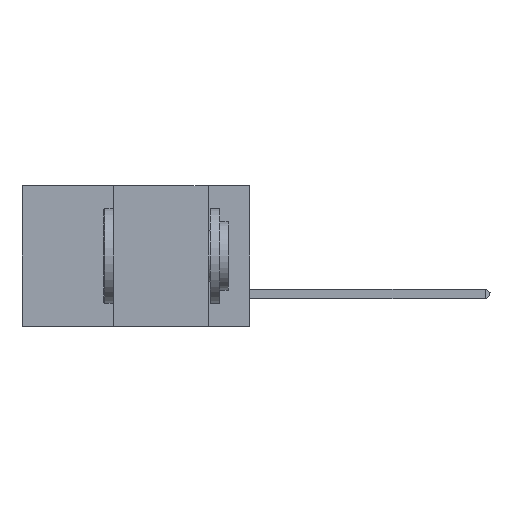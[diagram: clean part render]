
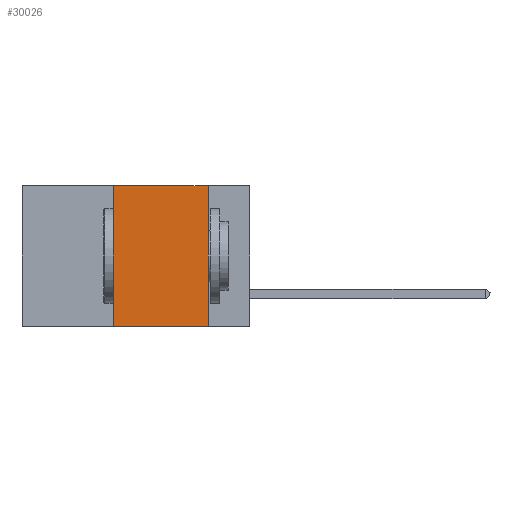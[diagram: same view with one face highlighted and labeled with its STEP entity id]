
A CAD part, left-side view. The second image highlights one B-rep face of the part: STEP entity #30026.
In plain terms, the highlighted planar face has unit normal (-1, 0, 0).
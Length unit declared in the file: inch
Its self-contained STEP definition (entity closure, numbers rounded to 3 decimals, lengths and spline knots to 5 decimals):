
#907 = ORIENTED_EDGE ( 'NONE', *, *, #15480, .F. ) ;
#1409 = CARTESIAN_POINT ( 'NONE',  ( 0., 0.6, 0. ) ) ;
#3148 = EDGE_LOOP ( 'NONE', ( #20717, #907, #8557, #7849 ) ) ;
#3651 = DIRECTION ( 'NONE',  ( 0., -1., 0. ) ) ;
#6938 = EDGE_CURVE ( 'NONE', #30591, #9729, #8733, .T. ) ;
#7202 = DIRECTION ( 'NONE',  ( 0., 0., -1. ) ) ;
#7849 = ORIENTED_EDGE ( 'NONE', *, *, #29242, .T. ) ;
#8557 = ORIENTED_EDGE ( 'NONE', *, *, #24955, .F. ) ;
#8733 = LINE ( 'NONE', #21648, #27178 ) ;
#9594 = CARTESIAN_POINT ( 'NONE',  ( 0., 0.36, 0. ) ) ;
#9729 = VERTEX_POINT ( 'NONE', #26616 ) ;
#11314 = LINE ( 'NONE', #15739, #28968 ) ;
#11721 = VERTEX_POINT ( 'NONE', #26762 ) ;
#12534 = VECTOR ( 'NONE', #13154, 39.37008 ) ;
#13154 = DIRECTION ( 'NONE',  ( 0., -1., 0. ) ) ;
#13181 = LINE ( 'NONE', #9594, #18786 ) ;
#15480 = EDGE_CURVE ( 'NONE', #11721, #30591, #25408, .T. ) ;
#15739 = CARTESIAN_POINT ( 'NONE',  ( 0., 0.6, -0.37 ) ) ;
#17217 = CARTESIAN_POINT ( 'NONE',  ( 0., 0.11, 0. ) ) ;
#18786 = VECTOR ( 'NONE', #24303, 39.37008 ) ;
#19504 = PLANE ( 'NONE',  #28611 ) ;
#20717 = ORIENTED_EDGE ( 'NONE', *, *, #6938, .F. ) ;
#21648 = CARTESIAN_POINT ( 'NONE',  ( 0., 0.11, 0. ) ) ;
#22063 = CARTESIAN_POINT ( 'NONE',  ( 0., 0.6, 0. ) ) ;
#22605 = FACE_OUTER_BOUND ( 'NONE', #3148, .T. ) ;
#24303 = DIRECTION ( 'NONE',  ( 0., 0., 1. ) ) ;
#24955 = EDGE_CURVE ( 'NONE', #28626, #11721, #13181, .T. ) ;
#25408 = LINE ( 'NONE', #1409, #12534 ) ;
#25671 = CARTESIAN_POINT ( 'NONE',  ( 0., 0.36, -0.37 ) ) ;
#26616 = CARTESIAN_POINT ( 'NONE',  ( 0., 0.11, -0.37 ) ) ;
#26762 = CARTESIAN_POINT ( 'NONE',  ( 0., 0.36, 0. ) ) ;
#27178 = VECTOR ( 'NONE', #7202, 39.37008 ) ;
#27220 = DIRECTION ( 'NONE',  ( 0., 0., -1. ) ) ;
#27325 = DIRECTION ( 'NONE',  ( 1., 0., 0. ) ) ;
#28611 = AXIS2_PLACEMENT_3D ( 'NONE', #22063, #27325, #27220 ) ;
#28626 = VERTEX_POINT ( 'NONE', #25671 ) ;
#28968 = VECTOR ( 'NONE', #3651, 39.37008 ) ;
#29242 = EDGE_CURVE ( 'NONE', #28626, #9729, #11314, .T. ) ;
#30026 = ADVANCED_FACE ( 'NONE', ( #22605 ), #19504, .F. ) ;
#30591 = VERTEX_POINT ( 'NONE', #17217 ) ;
